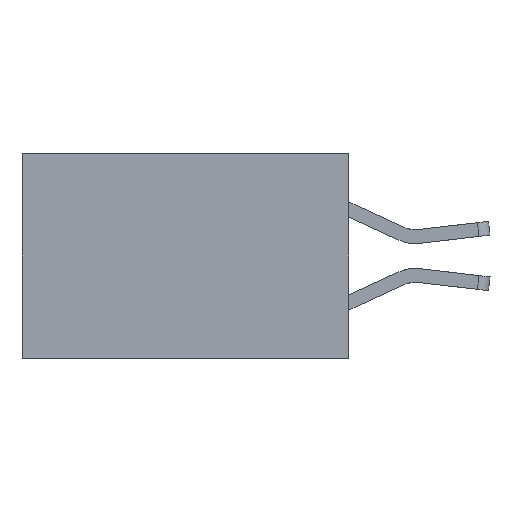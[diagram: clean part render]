
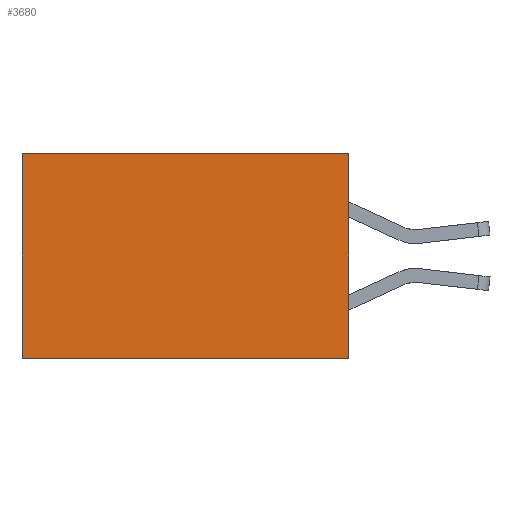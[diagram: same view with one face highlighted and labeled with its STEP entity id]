
A CAD part, left-side view. The second image highlights one B-rep face of the part: STEP entity #3680.
In plain terms, the highlighted planar face has unit normal (-1, 0, 0).
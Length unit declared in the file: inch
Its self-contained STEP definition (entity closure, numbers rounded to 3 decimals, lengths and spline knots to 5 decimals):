
#323 = EDGE_CURVE ( 'NONE', #6952, #6678, #4624, .T. ) ;
#388 = LINE ( 'NONE', #3315, #1854 ) ;
#673 = VERTEX_POINT ( 'NONE', #4615 ) ;
#1103 = EDGE_LOOP ( 'NONE', ( #6611, #3530, #2256, #7252 ) ) ;
#1418 = EDGE_CURVE ( 'NONE', #2064, #6952, #3299, .T. ) ;
#1591 = VECTOR ( 'NONE', #2342, 39.37008 ) ;
#1644 = CARTESIAN_POINT ( 'NONE',  ( 0.277, 0.59, 0. ) ) ;
#1825 = CARTESIAN_POINT ( 'NONE',  ( 0.277, 0.59, -0.37 ) ) ;
#1854 = VECTOR ( 'NONE', #3636, 39.37008 ) ;
#1867 = FACE_OUTER_BOUND ( 'NONE', #1103, .T. ) ;
#2064 = VERTEX_POINT ( 'NONE', #3072 ) ;
#2236 = CARTESIAN_POINT ( 'NONE',  ( 0.277, 0., 0. ) ) ;
#2256 = ORIENTED_EDGE ( 'NONE', *, *, #4162, .F. ) ;
#2342 = DIRECTION ( 'NONE',  ( 0., 1., 0. ) ) ;
#3072 = CARTESIAN_POINT ( 'NONE',  ( 0.277, 0., 0. ) ) ;
#3299 = LINE ( 'NONE', #2236, #1591 ) ;
#3315 = CARTESIAN_POINT ( 'NONE',  ( 0.277, 0., -0.37 ) ) ;
#3530 = ORIENTED_EDGE ( 'NONE', *, *, #4105, .F. ) ;
#3636 = DIRECTION ( 'NONE',  ( 0., 0., -1. ) ) ;
#3667 = DIRECTION ( 'NONE',  ( 0., 0., -1. ) ) ;
#3680 = ADVANCED_FACE ( 'NONE', ( #1867 ), #7675, .F. ) ;
#3762 = AXIS2_PLACEMENT_3D ( 'NONE', #7638, #7179, #7615 ) ;
#3913 = VECTOR ( 'NONE', #4176, 39.37008 ) ;
#4105 = EDGE_CURVE ( 'NONE', #673, #6678, #6156, .T. ) ;
#4162 = EDGE_CURVE ( 'NONE', #2064, #673, #388, .T. ) ;
#4176 = DIRECTION ( 'NONE',  ( 0., 1., 0. ) ) ;
#4615 = CARTESIAN_POINT ( 'NONE',  ( 0.277, 0., -0.37 ) ) ;
#4624 = LINE ( 'NONE', #1825, #7239 ) ;
#4712 = CARTESIAN_POINT ( 'NONE',  ( 0.277, 0., -0.37 ) ) ;
#5262 = CARTESIAN_POINT ( 'NONE',  ( 0.277, 0.59, -0.37 ) ) ;
#6156 = LINE ( 'NONE', #4712, #3913 ) ;
#6611 = ORIENTED_EDGE ( 'NONE', *, *, #323, .T. ) ;
#6678 = VERTEX_POINT ( 'NONE', #5262 ) ;
#6952 = VERTEX_POINT ( 'NONE', #1644 ) ;
#7179 = DIRECTION ( 'NONE',  ( 1., 0., 0. ) ) ;
#7239 = VECTOR ( 'NONE', #3667, 39.37008 ) ;
#7252 = ORIENTED_EDGE ( 'NONE', *, *, #1418, .T. ) ;
#7615 = DIRECTION ( 'NONE',  ( 0., 0., -1. ) ) ;
#7638 = CARTESIAN_POINT ( 'NONE',  ( 0.277, 0., -0.37 ) ) ;
#7675 = PLANE ( 'NONE',  #3762 ) ;
